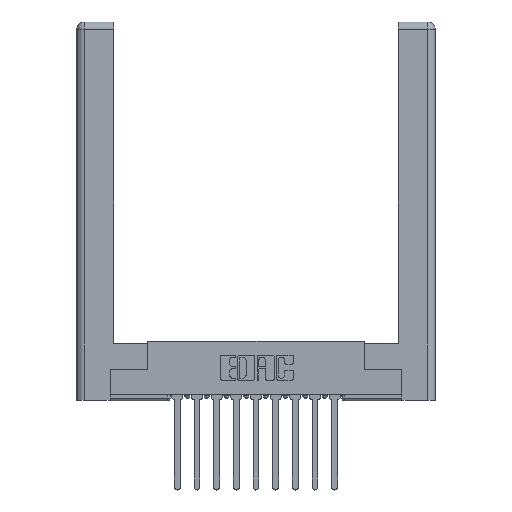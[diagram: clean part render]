
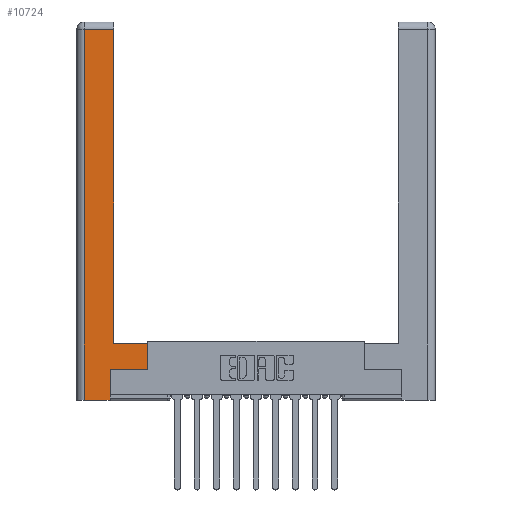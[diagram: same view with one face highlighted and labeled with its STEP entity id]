
A CAD part, top view. The second image highlights one B-rep face of the part: STEP entity #10724.
In plain terms, the highlighted planar face has unit normal (0, 0, 1).
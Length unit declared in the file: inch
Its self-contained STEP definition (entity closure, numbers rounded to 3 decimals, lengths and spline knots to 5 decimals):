
#1114 = VERTEX_POINT ( 'NONE', #5043 ) ;
#1366 = CARTESIAN_POINT ( 'NONE',  ( 0.0615, 0., 0. ) ) ;
#1565 = DIRECTION ( 'NONE',  ( 0., 1., 0. ) ) ;
#1702 = CARTESIAN_POINT ( 'NONE',  ( 0.295, 0.45, 0. ) ) ;
#2116 = ORIENTED_EDGE ( 'NONE', *, *, #13105, .T. ) ;
#2339 = CARTESIAN_POINT ( 'NONE',  ( 0.565, 0.245, 0. ) ) ;
#2395 = AXIS2_PLACEMENT_3D ( 'NONE', #8008, #10228, #13658 ) ;
#2819 = DIRECTION ( 'NONE',  ( 1., 0., 0. ) ) ;
#2925 = DIRECTION ( 'NONE',  ( -1., 0., 0. ) ) ;
#3150 = DIRECTION ( 'NONE',  ( 0., 1., 0. ) ) ;
#3291 = DIRECTION ( 'NONE',  ( 0., 1., 0. ) ) ;
#3301 = ORIENTED_EDGE ( 'NONE', *, *, #10019, .T. ) ;
#3603 = VECTOR ( 'NONE', #3687, 39.37008 ) ;
#3635 = CARTESIAN_POINT ( 'NONE',  ( 0.565, 0.245, 0. ) ) ;
#3687 = DIRECTION ( 'NONE',  ( 0., -1., 0. ) ) ;
#4455 = ORIENTED_EDGE ( 'NONE', *, *, #14216, .T. ) ;
#4521 = ORIENTED_EDGE ( 'NONE', *, *, #6750, .T. ) ;
#5043 = CARTESIAN_POINT ( 'NONE',  ( 0.565, 0.45, 0. ) ) ;
#5145 = CARTESIAN_POINT ( 'NONE',  ( 0.0615, 2.94, 0. ) ) ;
#5274 = VECTOR ( 'NONE', #3291, 39.37008 ) ;
#6385 = VECTOR ( 'NONE', #2925, 39.37008 ) ;
#6563 = EDGE_CURVE ( 'NONE', #7700, #1114, #7362, .T. ) ;
#6750 = EDGE_CURVE ( 'NONE', #9700, #10764, #14502, .T. ) ;
#6818 = PLANE ( 'NONE',  #2395 ) ;
#6885 = ORIENTED_EDGE ( 'NONE', *, *, #13896, .T. ) ;
#7265 = VECTOR ( 'NONE', #1565, 39.37008 ) ;
#7330 = LINE ( 'NONE', #3635, #8111 ) ;
#7339 = ORIENTED_EDGE ( 'NONE', *, *, #11990, .T. ) ;
#7347 = DIRECTION ( 'NONE',  ( -1., 0., 0. ) ) ;
#7362 = LINE ( 'NONE', #13905, #7265 ) ;
#7363 = LINE ( 'NONE', #5145, #6385 ) ;
#7411 = VECTOR ( 'NONE', #7347, 39.37008 ) ;
#7603 = CARTESIAN_POINT ( 'NONE',  ( 0.295, 0.45, 0. ) ) ;
#7700 = VERTEX_POINT ( 'NONE', #2339 ) ;
#8008 = CARTESIAN_POINT ( 'NONE',  ( 0., 0., 0. ) ) ;
#8111 = VECTOR ( 'NONE', #8158, 39.37008 ) ;
#8158 = DIRECTION ( 'NONE',  ( 1., 0., 0. ) ) ;
#8170 = ORIENTED_EDGE ( 'NONE', *, *, #6563, .T. ) ;
#8296 = CARTESIAN_POINT ( 'NONE',  ( 0.295, 2.94, 0. ) ) ;
#8768 = VERTEX_POINT ( 'NONE', #9948 ) ;
#8769 = CARTESIAN_POINT ( 'NONE',  ( 0.295, 3., 0. ) ) ;
#9135 = LINE ( 'NONE', #13679, #5274 ) ;
#9442 = CARTESIAN_POINT ( 'NONE',  ( 0.0615, 0., 0. ) ) ;
#9700 = VERTEX_POINT ( 'NONE', #7603 ) ;
#9948 = CARTESIAN_POINT ( 'NONE',  ( 0.265, 0.245, 0. ) ) ;
#10019 = EDGE_CURVE ( 'NONE', #10764, #11030, #7363, .T. ) ;
#10137 = LINE ( 'NONE', #1366, #3603 ) ;
#10194 = CARTESIAN_POINT ( 'NONE',  ( 0.0615, 2.94, 0. ) ) ;
#10228 = DIRECTION ( 'NONE',  ( 0., 0., -1. ) ) ;
#10724 = ADVANCED_FACE ( 'NONE', ( #12462 ), #6818, .F. ) ;
#10764 = VERTEX_POINT ( 'NONE', #8296 ) ;
#10977 = VECTOR ( 'NONE', #2819, 39.37008 ) ;
#11030 = VERTEX_POINT ( 'NONE', #10194 ) ;
#11049 = CARTESIAN_POINT ( 'NONE',  ( 0.265, 0., 0. ) ) ;
#11068 = LINE ( 'NONE', #1702, #7411 ) ;
#11075 = VECTOR ( 'NONE', #3150, 39.37008 ) ;
#11244 = VERTEX_POINT ( 'NONE', #9442 ) ;
#11990 = EDGE_CURVE ( 'NONE', #8768, #7700, #7330, .T. ) ;
#12075 = CARTESIAN_POINT ( 'NONE',  ( 0.265, 0., 0. ) ) ;
#12462 = FACE_OUTER_BOUND ( 'NONE', #14585, .T. ) ;
#12860 = ORIENTED_EDGE ( 'NONE', *, *, #14669, .T. ) ;
#13078 = VERTEX_POINT ( 'NONE', #11049 ) ;
#13105 = EDGE_CURVE ( 'NONE', #11030, #11244, #10137, .T. ) ;
#13658 = DIRECTION ( 'NONE',  ( -1., 0., 0. ) ) ;
#13679 = CARTESIAN_POINT ( 'NONE',  ( 0.265, 0.245, 0. ) ) ;
#13896 = EDGE_CURVE ( 'NONE', #13078, #8768, #9135, .T. ) ;
#13905 = CARTESIAN_POINT ( 'NONE',  ( 0.565, 0.45, 0. ) ) ;
#14098 = LINE ( 'NONE', #12075, #10977 ) ;
#14216 = EDGE_CURVE ( 'NONE', #1114, #9700, #11068, .T. ) ;
#14502 = LINE ( 'NONE', #8769, #11075 ) ;
#14585 = EDGE_LOOP ( 'NONE', ( #4521, #3301, #2116, #12860, #6885, #7339, #8170, #4455 ) ) ;
#14669 = EDGE_CURVE ( 'NONE', #11244, #13078, #14098, .T. ) ;
